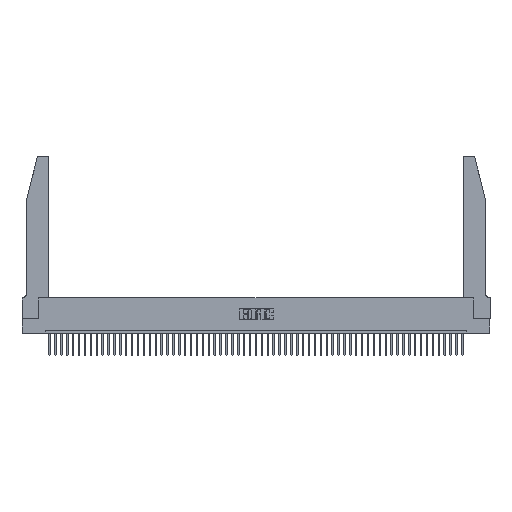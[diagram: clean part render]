
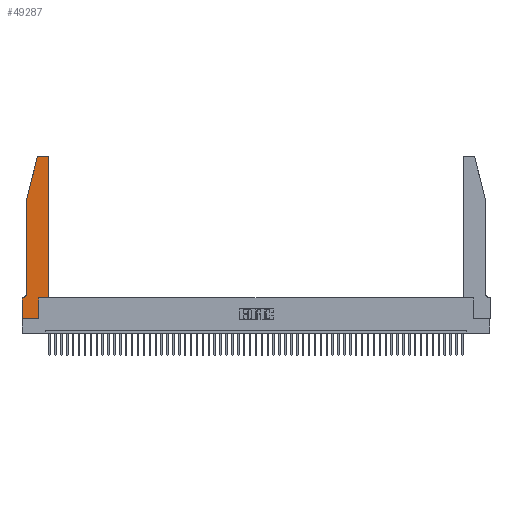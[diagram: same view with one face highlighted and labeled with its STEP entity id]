
A CAD part, top view. The second image highlights one B-rep face of the part: STEP entity #49287.
In plain terms, the highlighted planar face has unit normal (0, 0, 1).
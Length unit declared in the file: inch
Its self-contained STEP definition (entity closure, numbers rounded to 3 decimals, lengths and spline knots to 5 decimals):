
#86 = CIRCLE ( 'NONE', #27639, 0.03 ) ;
#143 = VERTEX_POINT ( 'NONE', #36637 ) ;
#426 = LINE ( 'NONE', #30706, #46957 ) ;
#1243 = DIRECTION ( 'NONE',  ( -1., 0., 0. ) ) ;
#1244 = LINE ( 'NONE', #41128, #13826 ) ;
#2071 = VERTEX_POINT ( 'NONE', #31820 ) ;
#2699 = DIRECTION ( 'NONE',  ( 0., 0., 1. ) ) ;
#3066 = ORIENTED_EDGE ( 'NONE', *, *, #53942, .T. ) ;
#3255 = ORIENTED_EDGE ( 'NONE', *, *, #40292, .T. ) ;
#4066 = DIRECTION ( 'NONE',  ( 1., 0., 0. ) ) ;
#4420 = VERTEX_POINT ( 'NONE', #20567 ) ;
#5057 = LINE ( 'NONE', #50777, #52239 ) ;
#5837 = EDGE_CURVE ( 'NONE', #8608, #143, #50724, .T. ) ;
#6233 = CARTESIAN_POINT ( 'NONE',  ( 0.284, 2.72, 0.37 ) ) ;
#6836 = DIRECTION ( 'NONE',  ( -1., 0., 0. ) ) ;
#6895 = FACE_OUTER_BOUND ( 'NONE', #26075, .T. ) ;
#8060 = ORIENTED_EDGE ( 'NONE', *, *, #34513, .T. ) ;
#8285 = EDGE_CURVE ( 'NONE', #35161, #45173, #11664, .T. ) ;
#8302 = VERTEX_POINT ( 'NONE', #15139 ) ;
#8608 = VERTEX_POINT ( 'NONE', #12646 ) ;
#9462 = CARTESIAN_POINT ( 'NONE',  ( 0.0055, 0.42, 0.37 ) ) ;
#10749 = LINE ( 'NONE', #26232, #19986 ) ;
#11379 = DIRECTION ( 'NONE',  ( 1., 0., 0. ) ) ;
#11506 = ORIENTED_EDGE ( 'NONE', *, *, #34533, .T. ) ;
#11664 = LINE ( 'NONE', #38728, #29947 ) ;
#11948 = VECTOR ( 'NONE', #6836, 39.37008 ) ;
#12257 = CARTESIAN_POINT ( 'NONE',  ( 0., 0.35, 0.37 ) ) ;
#12646 = CARTESIAN_POINT ( 'NONE',  ( 0.4505, 0.35, 0.37 ) ) ;
#13826 = VECTOR ( 'NONE', #30236, 39.37008 ) ;
#14955 = CARTESIAN_POINT ( 'NONE',  ( 0., 0., 0.37 ) ) ;
#15139 = CARTESIAN_POINT ( 'NONE',  ( 0.0055, 0.35, 0.37 ) ) ;
#15325 = VECTOR ( 'NONE', #43498, 39.37008 ) ;
#16992 = ORIENTED_EDGE ( 'NONE', *, *, #28604, .T. ) ;
#17634 = ORIENTED_EDGE ( 'NONE', *, *, #28977, .T. ) ;
#17725 = ORIENTED_EDGE ( 'NONE', *, *, #38982, .T. ) ;
#17741 = AXIS2_PLACEMENT_3D ( 'NONE', #53326, #2699, #11379 ) ;
#18177 = DIRECTION ( 'NONE',  ( 0., 0., -1. ) ) ;
#18419 = VERTEX_POINT ( 'NONE', #50033 ) ;
#19014 = CARTESIAN_POINT ( 'NONE',  ( 0.2605, 2.75, 0.37 ) ) ;
#19203 = CIRCLE ( 'NONE', #33109, 0.07 ) ;
#19562 = CARTESIAN_POINT ( 'NONE',  ( 0.0755, 0.42, 0.37 ) ) ;
#19632 = ORIENTED_EDGE ( 'NONE', *, *, #5837, .T. ) ;
#19756 = LINE ( 'NONE', #19014, #11948 ) ;
#19828 = DIRECTION ( 'NONE',  ( 1., 0., 0. ) ) ;
#19986 = VECTOR ( 'NONE', #24993, 39.37008 ) ;
#20567 = CARTESIAN_POINT ( 'NONE',  ( 0.0755, 2., 0.37 ) ) ;
#21282 = ORIENTED_EDGE ( 'NONE', *, *, #42193, .T. ) ;
#24219 = VERTEX_POINT ( 'NONE', #19562 ) ;
#24993 = DIRECTION ( 'NONE',  ( -1., 0., 0. ) ) ;
#25041 = VERTEX_POINT ( 'NONE', #44545 ) ;
#25513 = VERTEX_POINT ( 'NONE', #35080 ) ;
#26075 = EDGE_LOOP ( 'NONE', ( #11506, #8060, #16992, #3255, #17725, #31446, #21282, #44632, #17634, #50663, #19632, #3066 ) ) ;
#26232 = CARTESIAN_POINT ( 'NONE',  ( 0.0755, 0.35, 0.37 ) ) ;
#27639 = AXIS2_PLACEMENT_3D ( 'NONE', #6233, #43579, #48169 ) ;
#28604 = EDGE_CURVE ( 'NONE', #18419, #4420, #426, .T. ) ;
#28813 = CARTESIAN_POINT ( 'NONE',  ( 0.2865, 0.35, 0.37 ) ) ;
#28977 = EDGE_CURVE ( 'NONE', #45173, #25513, #34726, .T. ) ;
#29947 = VECTOR ( 'NONE', #42818, 39.37008 ) ;
#30236 = DIRECTION ( 'NONE',  ( 0., -1., 0. ) ) ;
#30706 = CARTESIAN_POINT ( 'NONE',  ( 0.0755, 2., 0.37 ) ) ;
#31446 = ORIENTED_EDGE ( 'NONE', *, *, #54092, .T. ) ;
#31820 = CARTESIAN_POINT ( 'NONE',  ( 0.284, 2.75, 0.37 ) ) ;
#33109 = AXIS2_PLACEMENT_3D ( 'NONE', #9462, #18177, #1243 ) ;
#34513 = EDGE_CURVE ( 'NONE', #2071, #18419, #86, .T. ) ;
#34533 = EDGE_CURVE ( 'NONE', #25041, #2071, #19756, .T. ) ;
#34660 = CARTESIAN_POINT ( 'NONE',  ( 0.2865, 0., 0.37 ) ) ;
#34726 = LINE ( 'NONE', #28813, #51699 ) ;
#35080 = CARTESIAN_POINT ( 'NONE',  ( 0.2865, 0.35, 0.37 ) ) ;
#35161 = VERTEX_POINT ( 'NONE', #14955 ) ;
#35809 = VERTEX_POINT ( 'NONE', #12257 ) ;
#36637 = CARTESIAN_POINT ( 'NONE',  ( 0.4505, 2.72, 0.37 ) ) ;
#37268 = DIRECTION ( 'NONE',  ( 0., 0., 1. ) ) ;
#37579 = DIRECTION ( 'NONE',  ( 0., 1., 0. ) ) ;
#38728 = CARTESIAN_POINT ( 'NONE',  ( 0., 0., 0.37 ) ) ;
#38773 = AXIS2_PLACEMENT_3D ( 'NONE', #41435, #37268, #4066 ) ;
#38982 = EDGE_CURVE ( 'NONE', #24219, #8302, #19203, .T. ) ;
#39287 = CARTESIAN_POINT ( 'NONE',  ( 0.4505, 0.35, 0.37 ) ) ;
#40292 = EDGE_CURVE ( 'NONE', #4420, #24219, #1244, .T. ) ;
#40416 = VECTOR ( 'NONE', #19828, 39.37008 ) ;
#41128 = CARTESIAN_POINT ( 'NONE',  ( 0.0755, 2., 0.37 ) ) ;
#41435 = CARTESIAN_POINT ( 'NONE',  ( 0.4205, 2.72, 0.37 ) ) ;
#41753 = LINE ( 'NONE', #52799, #40416 ) ;
#42193 = EDGE_CURVE ( 'NONE', #35809, #35161, #5057, .T. ) ;
#42746 = EDGE_CURVE ( 'NONE', #25513, #8608, #41753, .T. ) ;
#42818 = DIRECTION ( 'NONE',  ( 1., 0., 0. ) ) ;
#42880 = CIRCLE ( 'NONE', #38773, 0.03 ) ;
#43115 = DIRECTION ( 'NONE',  ( -0.239, -0.971, 0. ) ) ;
#43498 = DIRECTION ( 'NONE',  ( 0., 1., 0. ) ) ;
#43579 = DIRECTION ( 'NONE',  ( 0., 0., 1. ) ) ;
#44545 = CARTESIAN_POINT ( 'NONE',  ( 0.4205, 2.75, 0.37 ) ) ;
#44632 = ORIENTED_EDGE ( 'NONE', *, *, #8285, .T. ) ;
#45173 = VERTEX_POINT ( 'NONE', #34660 ) ;
#46957 = VECTOR ( 'NONE', #43115, 39.37008 ) ;
#48169 = DIRECTION ( 'NONE',  ( 1., 0., 0. ) ) ;
#49287 = ADVANCED_FACE ( 'NONE', ( #6895 ), #53706, .T. ) ;
#49344 = DIRECTION ( 'NONE',  ( 0., -1., 0. ) ) ;
#50033 = CARTESIAN_POINT ( 'NONE',  ( 0.25487, 2.72718, 0.37 ) ) ;
#50663 = ORIENTED_EDGE ( 'NONE', *, *, #42746, .T. ) ;
#50724 = LINE ( 'NONE', #39287, #15325 ) ;
#50777 = CARTESIAN_POINT ( 'NONE',  ( 0., 0., 0.37 ) ) ;
#51699 = VECTOR ( 'NONE', #37579, 39.37008 ) ;
#52239 = VECTOR ( 'NONE', #49344, 39.37008 ) ;
#52799 = CARTESIAN_POINT ( 'NONE',  ( 0.4505, 0.35, 0.37 ) ) ;
#53326 = CARTESIAN_POINT ( 'NONE',  ( 0., 0.35, 0.37 ) ) ;
#53706 = PLANE ( 'NONE',  #17741 ) ;
#53942 = EDGE_CURVE ( 'NONE', #143, #25041, #42880, .T. ) ;
#54092 = EDGE_CURVE ( 'NONE', #8302, #35809, #10749, .T. ) ;
